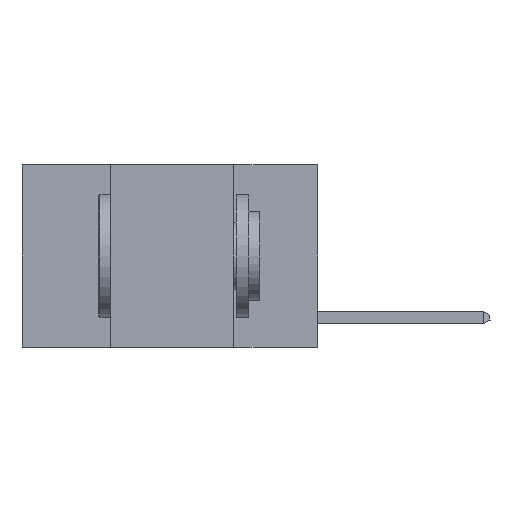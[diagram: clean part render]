
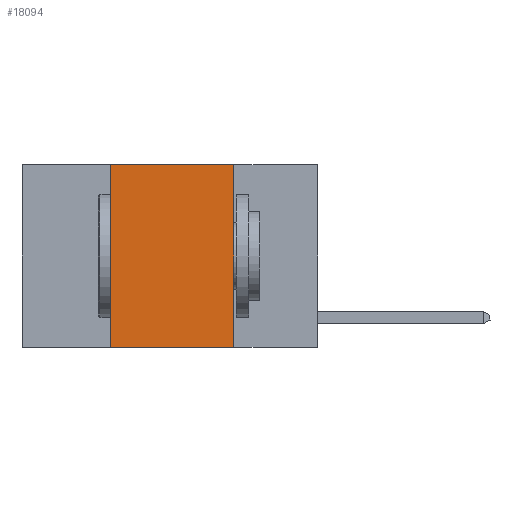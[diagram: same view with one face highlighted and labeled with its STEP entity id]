
A CAD part, left-side view. The second image highlights one B-rep face of the part: STEP entity #18094.
In plain terms, the highlighted planar face has unit normal (-1, 0, 0).
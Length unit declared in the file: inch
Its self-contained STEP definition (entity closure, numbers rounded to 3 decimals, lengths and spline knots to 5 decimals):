
#118 = ORIENTED_EDGE ( 'NONE', *, *, #15765, .F. ) ;
#678 = CARTESIAN_POINT ( 'NONE',  ( 0., 0.6, 0. ) ) ;
#1017 = VERTEX_POINT ( 'NONE', #2975 ) ;
#2181 = DIRECTION ( 'NONE',  ( 1., 0., 0. ) ) ;
#2699 = ORIENTED_EDGE ( 'NONE', *, *, #5901, .T. ) ;
#2975 = CARTESIAN_POINT ( 'NONE',  ( 0., 0.42, -0.37 ) ) ;
#3022 = LINE ( 'NONE', #17427, #18202 ) ;
#3545 = ORIENTED_EDGE ( 'NONE', *, *, #14505, .F. ) ;
#4272 = DIRECTION ( 'NONE',  ( 0., -1., 0. ) ) ;
#4310 = LINE ( 'NONE', #17504, #15601 ) ;
#5136 = DIRECTION ( 'NONE',  ( 0., 0., 1. ) ) ;
#5901 = EDGE_CURVE ( 'NONE', #1017, #16997, #14535, .T. ) ;
#6427 = DIRECTION ( 'NONE',  ( 0., -1., 0. ) ) ;
#7303 = EDGE_CURVE ( 'NONE', #10990, #16997, #4310, .T. ) ;
#8801 = LINE ( 'NONE', #15410, #9266 ) ;
#9266 = VECTOR ( 'NONE', #5136, 39.37008 ) ;
#9409 = CARTESIAN_POINT ( 'NONE',  ( 0., 0.6, -0.37 ) ) ;
#9602 = PLANE ( 'NONE',  #16843 ) ;
#10670 = EDGE_LOOP ( 'NONE', ( #11059, #3545, #118, #2699 ) ) ;
#10990 = VERTEX_POINT ( 'NONE', #11495 ) ;
#11059 = ORIENTED_EDGE ( 'NONE', *, *, #7303, .F. ) ;
#11495 = CARTESIAN_POINT ( 'NONE',  ( 0., 0.17, 0. ) ) ;
#12532 = CARTESIAN_POINT ( 'NONE',  ( 0., 0.17, -0.37 ) ) ;
#12599 = DIRECTION ( 'NONE',  ( 0., 0., -1. ) ) ;
#12966 = CARTESIAN_POINT ( 'NONE',  ( 0., 0.42, 0. ) ) ;
#14425 = VERTEX_POINT ( 'NONE', #12966 ) ;
#14505 = EDGE_CURVE ( 'NONE', #14425, #10990, #3022, .T. ) ;
#14535 = LINE ( 'NONE', #9409, #17907 ) ;
#15410 = CARTESIAN_POINT ( 'NONE',  ( 0., 0.42, 0. ) ) ;
#15601 = VECTOR ( 'NONE', #18963, 39.37008 ) ;
#15765 = EDGE_CURVE ( 'NONE', #1017, #14425, #8801, .T. ) ;
#16722 = FACE_OUTER_BOUND ( 'NONE', #10670, .T. ) ;
#16843 = AXIS2_PLACEMENT_3D ( 'NONE', #678, #2181, #12599 ) ;
#16997 = VERTEX_POINT ( 'NONE', #12532 ) ;
#17427 = CARTESIAN_POINT ( 'NONE',  ( 0., 0.6, 0. ) ) ;
#17504 = CARTESIAN_POINT ( 'NONE',  ( 0., 0.17, 0. ) ) ;
#17907 = VECTOR ( 'NONE', #6427, 39.37008 ) ;
#18094 = ADVANCED_FACE ( 'NONE', ( #16722 ), #9602, .F. ) ;
#18202 = VECTOR ( 'NONE', #4272, 39.37008 ) ;
#18963 = DIRECTION ( 'NONE',  ( 0., 0., -1. ) ) ;
